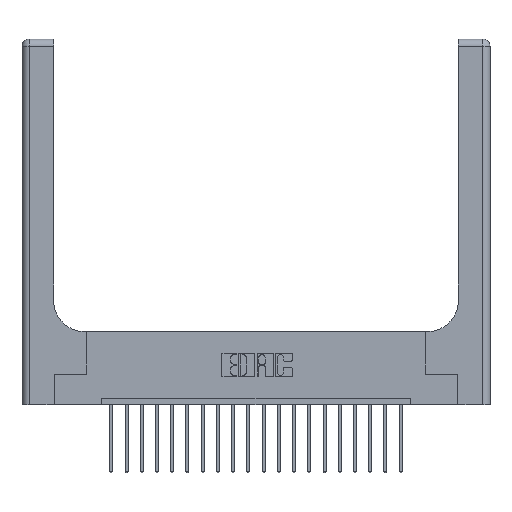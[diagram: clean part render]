
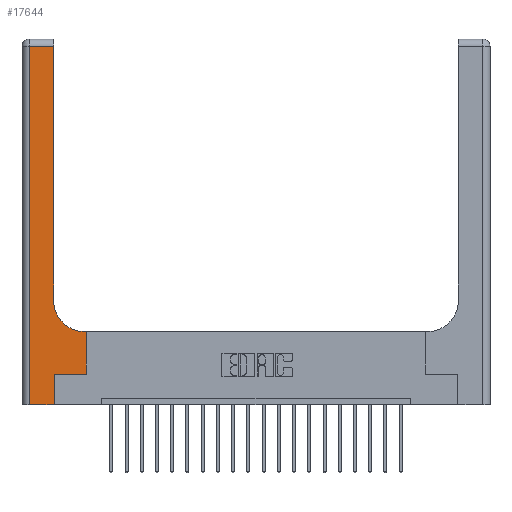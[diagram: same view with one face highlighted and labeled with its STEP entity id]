
A CAD part, top view. The second image highlights one B-rep face of the part: STEP entity #17644.
In plain terms, the highlighted planar face has unit normal (0, 0, 1).
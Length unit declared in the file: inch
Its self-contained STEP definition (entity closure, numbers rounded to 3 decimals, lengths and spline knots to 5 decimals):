
#98 = LINE ( 'NONE', #4516, #2364 ) ;
#816 = EDGE_CURVE ( 'NONE', #15822, #19514, #10417, .T. ) ;
#975 = ORIENTED_EDGE ( 'NONE', *, *, #816, .T. ) ;
#1402 = EDGE_CURVE ( 'NONE', #13667, #15822, #4440, .T. ) ;
#1876 = CARTESIAN_POINT ( 'NONE',  ( 0.528, 0.25, 0.37 ) ) ;
#2019 = VECTOR ( 'NONE', #3479, 39.37008 ) ;
#2237 = DIRECTION ( 'NONE',  ( 1., 0., 0. ) ) ;
#2349 = DIRECTION ( 'NONE',  ( 0., 0., -1. ) ) ;
#2361 = VERTEX_POINT ( 'NONE', #14317 ) ;
#2364 = VECTOR ( 'NONE', #15772, 39.37008 ) ;
#2432 = VECTOR ( 'NONE', #14660, 39.37008 ) ;
#2443 = VECTOR ( 'NONE', #4219, 39.37008 ) ;
#2799 = DIRECTION ( 'NONE',  ( 1., 0., 0. ) ) ;
#3017 = AXIS2_PLACEMENT_3D ( 'NONE', #3961, #10178, #7177 ) ;
#3043 = DIRECTION ( 'NONE',  ( -1., 0., 0. ) ) ;
#3479 = DIRECTION ( 'NONE',  ( 0., 1., 0. ) ) ;
#3513 = CARTESIAN_POINT ( 'NONE',  ( 0.265, 0., 0.37 ) ) ;
#3748 = CARTESIAN_POINT ( 'NONE',  ( 0., 0., 0.37 ) ) ;
#3922 = EDGE_CURVE ( 'NONE', #14166, #13667, #98, .T. ) ;
#3961 = CARTESIAN_POINT ( 'NONE',  ( 0.51, 0.85, 0.37 ) ) ;
#4219 = DIRECTION ( 'NONE',  ( 0., -1., 0. ) ) ;
#4440 = LINE ( 'NONE', #18525, #2443 ) ;
#4490 = DIRECTION ( 'NONE',  ( 0., 1., 0. ) ) ;
#4516 = CARTESIAN_POINT ( 'NONE',  ( 0., 2.94, 0.37 ) ) ;
#5058 = ORIENTED_EDGE ( 'NONE', *, *, #16539, .T. ) ;
#5126 = EDGE_LOOP ( 'NONE', ( #5058, #11710, #13108, #975, #7726, #11281, #8127, #19848, #14207 ) ) ;
#5216 = CARTESIAN_POINT ( 'NONE',  ( 0.26, 2.94, 0.37 ) ) ;
#5413 = LINE ( 'NONE', #12399, #9134 ) ;
#5795 = EDGE_CURVE ( 'NONE', #19514, #15365, #17847, .T. ) ;
#6323 = EDGE_CURVE ( 'NONE', #13613, #10157, #12355, .T. ) ;
#6937 = LINE ( 'NONE', #15558, #10432 ) ;
#7177 = DIRECTION ( 'NONE',  ( 1., 0., 0. ) ) ;
#7726 = ORIENTED_EDGE ( 'NONE', *, *, #5795, .T. ) ;
#8127 = ORIENTED_EDGE ( 'NONE', *, *, #14429, .T. ) ;
#9134 = VECTOR ( 'NONE', #4490, 39.37008 ) ;
#9848 = FACE_OUTER_BOUND ( 'NONE', #5126, .T. ) ;
#9860 = CARTESIAN_POINT ( 'NONE',  ( 0.265, 0., 0.37 ) ) ;
#10157 = VERTEX_POINT ( 'NONE', #12368 ) ;
#10178 = DIRECTION ( 'NONE',  ( 0., 0., -1. ) ) ;
#10417 = LINE ( 'NONE', #3748, #10926 ) ;
#10432 = VECTOR ( 'NONE', #3043, 39.37008 ) ;
#10736 = CARTESIAN_POINT ( 'NONE',  ( 0.528, 0.6, 0.37 ) ) ;
#10842 = EDGE_CURVE ( 'NONE', #14677, #13613, #6937, .T. ) ;
#10876 = VECTOR ( 'NONE', #2799, 39.37008 ) ;
#10926 = VECTOR ( 'NONE', #2237, 39.37008 ) ;
#11281 = ORIENTED_EDGE ( 'NONE', *, *, #17151, .T. ) ;
#11710 = ORIENTED_EDGE ( 'NONE', *, *, #3922, .T. ) ;
#12355 = CIRCLE ( 'NONE', #3017, 0.25 ) ;
#12368 = CARTESIAN_POINT ( 'NONE',  ( 0.26, 0.85, 0.37 ) ) ;
#12399 = CARTESIAN_POINT ( 'NONE',  ( 0.26, 3., 0.37 ) ) ;
#13108 = ORIENTED_EDGE ( 'NONE', *, *, #1402, .T. ) ;
#13601 = DIRECTION ( 'NONE',  ( -1., 0., 0. ) ) ;
#13613 = VERTEX_POINT ( 'NONE', #16084 ) ;
#13667 = VERTEX_POINT ( 'NONE', #15253 ) ;
#14166 = VERTEX_POINT ( 'NONE', #5216 ) ;
#14207 = ORIENTED_EDGE ( 'NONE', *, *, #6323, .T. ) ;
#14317 = CARTESIAN_POINT ( 'NONE',  ( 0.528, 0.25, 0.37 ) ) ;
#14429 = EDGE_CURVE ( 'NONE', #2361, #14677, #18677, .T. ) ;
#14660 = DIRECTION ( 'NONE',  ( 0., 1., 0. ) ) ;
#14677 = VERTEX_POINT ( 'NONE', #10736 ) ;
#15227 = CARTESIAN_POINT ( 'NONE',  ( 0., 3., 0.37 ) ) ;
#15253 = CARTESIAN_POINT ( 'NONE',  ( 0.06, 2.94, 0.37 ) ) ;
#15312 = CARTESIAN_POINT ( 'NONE',  ( 0.265, 0.25, 0.37 ) ) ;
#15365 = VERTEX_POINT ( 'NONE', #20340 ) ;
#15558 = CARTESIAN_POINT ( 'NONE',  ( 0.26, 0.6, 0.37 ) ) ;
#15772 = DIRECTION ( 'NONE',  ( -1., 0., 0. ) ) ;
#15799 = AXIS2_PLACEMENT_3D ( 'NONE', #15227, #2349, #13601 ) ;
#15822 = VERTEX_POINT ( 'NONE', #18217 ) ;
#16084 = CARTESIAN_POINT ( 'NONE',  ( 0.51, 0.6, 0.37 ) ) ;
#16539 = EDGE_CURVE ( 'NONE', #10157, #14166, #5413, .T. ) ;
#17151 = EDGE_CURVE ( 'NONE', #15365, #2361, #20279, .T. ) ;
#17644 = ADVANCED_FACE ( 'NONE', ( #9848 ), #18330, .F. ) ;
#17847 = LINE ( 'NONE', #3513, #2432 ) ;
#18217 = CARTESIAN_POINT ( 'NONE',  ( 0.06, 0., 0.37 ) ) ;
#18330 = PLANE ( 'NONE',  #15799 ) ;
#18525 = CARTESIAN_POINT ( 'NONE',  ( 0.06, 3., 0.37 ) ) ;
#18677 = LINE ( 'NONE', #1876, #2019 ) ;
#19514 = VERTEX_POINT ( 'NONE', #9860 ) ;
#19848 = ORIENTED_EDGE ( 'NONE', *, *, #10842, .T. ) ;
#20279 = LINE ( 'NONE', #15312, #10876 ) ;
#20340 = CARTESIAN_POINT ( 'NONE',  ( 0.265, 0.25, 0.37 ) ) ;
